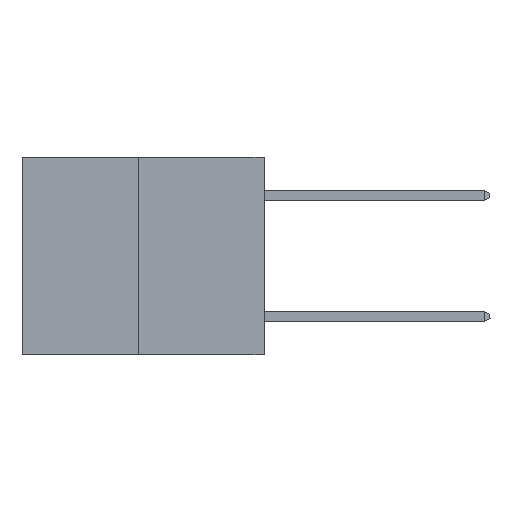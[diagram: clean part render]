
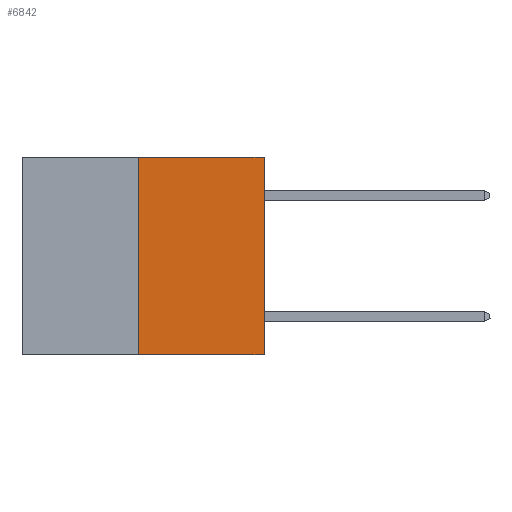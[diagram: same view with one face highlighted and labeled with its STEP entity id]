
A CAD part, left-side view. The second image highlights one B-rep face of the part: STEP entity #6842.
In plain terms, the highlighted planar face has unit normal (-1, 0, 0).
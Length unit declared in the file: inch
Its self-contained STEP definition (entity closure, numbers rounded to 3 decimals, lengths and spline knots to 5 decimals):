
#836 = EDGE_CURVE ( 'NONE', #15497, #11736, #3097, .T. ) ;
#1976 = VECTOR ( 'NONE', #19945, 39.37008 ) ;
#2551 = EDGE_CURVE ( 'NONE', #2940, #20911, #3059, .T. ) ;
#2801 = DIRECTION ( 'NONE',  ( 1., 0., 0. ) ) ;
#2940 = VERTEX_POINT ( 'NONE', #8343 ) ;
#3059 = LINE ( 'NONE', #11340, #1976 ) ;
#3097 = LINE ( 'NONE', #20645, #20742 ) ;
#3622 = EDGE_CURVE ( 'NONE', #15497, #2940, #21457, .T. ) ;
#3752 = VECTOR ( 'NONE', #12757, 39.37008 ) ;
#4127 = EDGE_CURVE ( 'NONE', #11736, #20911, #20875, .T. ) ;
#4134 = CARTESIAN_POINT ( 'NONE',  ( 0., 0., 0. ) ) ;
#4151 = ORIENTED_EDGE ( 'NONE', *, *, #4127, .T. ) ;
#4365 = CARTESIAN_POINT ( 'NONE',  ( 0., 0.6, 0. ) ) ;
#5301 = DIRECTION ( 'NONE',  ( 0., -1., 0. ) ) ;
#5409 = AXIS2_PLACEMENT_3D ( 'NONE', #4365, #2801, #16468 ) ;
#6842 = ADVANCED_FACE ( 'NONE', ( #19297 ), #7729, .F. ) ;
#7613 = EDGE_LOOP ( 'NONE', ( #14573, #16533, #4151, #19465 ) ) ;
#7729 = PLANE ( 'NONE',  #5409 ) ;
#8343 = CARTESIAN_POINT ( 'NONE',  ( 0., 0.312, 0. ) ) ;
#9577 = CARTESIAN_POINT ( 'NONE',  ( 0., 0.312, -0.49 ) ) ;
#11340 = CARTESIAN_POINT ( 'NONE',  ( 0., 0.6, 0. ) ) ;
#11736 = VERTEX_POINT ( 'NONE', #13295 ) ;
#12757 = DIRECTION ( 'NONE',  ( 0., 0., 1. ) ) ;
#13295 = CARTESIAN_POINT ( 'NONE',  ( 0., 0., -0.49 ) ) ;
#13430 = VECTOR ( 'NONE', #21332, 39.37008 ) ;
#14573 = ORIENTED_EDGE ( 'NONE', *, *, #3622, .F. ) ;
#15497 = VERTEX_POINT ( 'NONE', #9577 ) ;
#15691 = CARTESIAN_POINT ( 'NONE',  ( 0., 0.312, -0.49 ) ) ;
#16468 = DIRECTION ( 'NONE',  ( 0., 0., -1. ) ) ;
#16533 = ORIENTED_EDGE ( 'NONE', *, *, #836, .T. ) ;
#19198 = CARTESIAN_POINT ( 'NONE',  ( 0., 0., 0. ) ) ;
#19297 = FACE_OUTER_BOUND ( 'NONE', #7613, .T. ) ;
#19465 = ORIENTED_EDGE ( 'NONE', *, *, #2551, .F. ) ;
#19945 = DIRECTION ( 'NONE',  ( 0., -1., 0. ) ) ;
#20645 = CARTESIAN_POINT ( 'NONE',  ( 0., 0.6, -0.49 ) ) ;
#20742 = VECTOR ( 'NONE', #5301, 39.37008 ) ;
#20875 = LINE ( 'NONE', #4134, #3752 ) ;
#20911 = VERTEX_POINT ( 'NONE', #19198 ) ;
#21332 = DIRECTION ( 'NONE',  ( 0., 0., 1. ) ) ;
#21457 = LINE ( 'NONE', #15691, #13430 ) ;
